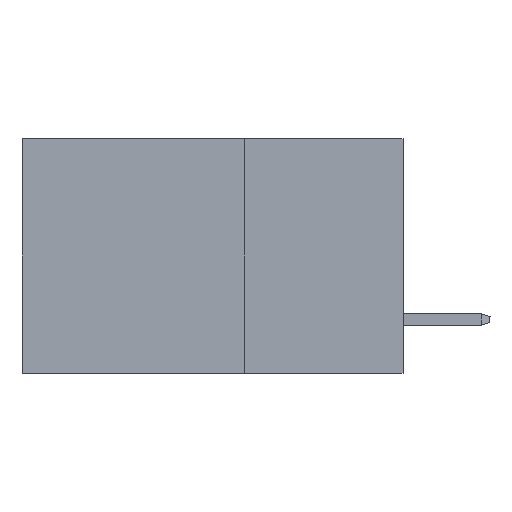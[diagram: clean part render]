
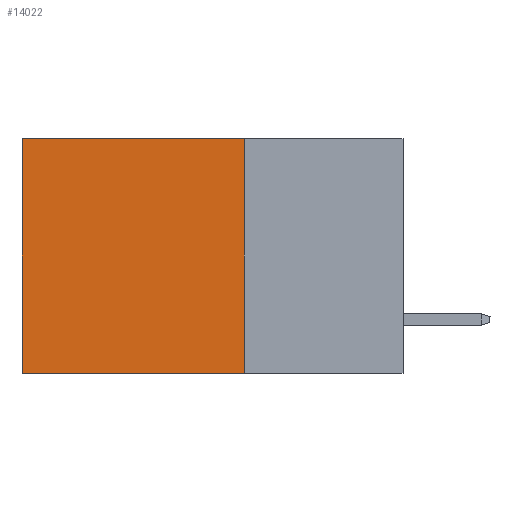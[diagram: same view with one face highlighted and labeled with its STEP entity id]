
A CAD part, left-side view. The second image highlights one B-rep face of the part: STEP entity #14022.
In plain terms, the highlighted planar face has unit normal (-1, 0, 0).
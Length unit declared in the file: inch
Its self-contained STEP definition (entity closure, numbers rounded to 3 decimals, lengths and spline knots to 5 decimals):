
#527 = VERTEX_POINT ( 'NONE', #16638 ) ;
#1776 = DIRECTION ( 'NONE',  ( 0., 0., -1. ) ) ;
#2168 = CARTESIAN_POINT ( 'NONE',  ( 0.2875, 0.6, 0. ) ) ;
#2653 = CARTESIAN_POINT ( 'NONE',  ( 0.2875, 0.25, 0. ) ) ;
#3952 = ORIENTED_EDGE ( 'NONE', *, *, #23253, .T. ) ;
#4387 = LINE ( 'NONE', #16398, #15092 ) ;
#6721 = DIRECTION ( 'NONE',  ( 1., 0., 0. ) ) ;
#6731 = DIRECTION ( 'NONE',  ( 0., 1., 0. ) ) ;
#7143 = DIRECTION ( 'NONE',  ( 0., 0., -1. ) ) ;
#7226 = CARTESIAN_POINT ( 'NONE',  ( 0.2875, 0.6, 0. ) ) ;
#8876 = LINE ( 'NONE', #11302, #16537 ) ;
#9631 = VECTOR ( 'NONE', #7143, 39.37008 ) ;
#9866 = EDGE_LOOP ( 'NONE', ( #25631, #18511, #17107, #3952 ) ) ;
#10125 = VECTOR ( 'NONE', #1776, 39.37008 ) ;
#11302 = CARTESIAN_POINT ( 'NONE',  ( 0.2875, 0.25, 0. ) ) ;
#11912 = VERTEX_POINT ( 'NONE', #24446 ) ;
#12943 = LINE ( 'NONE', #23744, #9631 ) ;
#13485 = EDGE_CURVE ( 'NONE', #18380, #527, #12943, .T. ) ;
#14022 = ADVANCED_FACE ( 'NONE', ( #25345 ), #16973, .F. ) ;
#14472 = LINE ( 'NONE', #2168, #10125 ) ;
#14944 = DIRECTION ( 'NONE',  ( 0., 0., -1. ) ) ;
#15092 = VECTOR ( 'NONE', #20857, 39.37008 ) ;
#15311 = AXIS2_PLACEMENT_3D ( 'NONE', #2653, #6721, #14944 ) ;
#16398 = CARTESIAN_POINT ( 'NONE',  ( 0.2875, 0.25, -0.37 ) ) ;
#16537 = VECTOR ( 'NONE', #6731, 39.37008 ) ;
#16638 = CARTESIAN_POINT ( 'NONE',  ( 0.2875, 0.25, -0.37 ) ) ;
#16973 = PLANE ( 'NONE',  #15311 ) ;
#17107 = ORIENTED_EDGE ( 'NONE', *, *, #13485, .F. ) ;
#17742 = EDGE_CURVE ( 'NONE', #527, #11912, #4387, .T. ) ;
#18380 = VERTEX_POINT ( 'NONE', #21088 ) ;
#18511 = ORIENTED_EDGE ( 'NONE', *, *, #17742, .F. ) ;
#20857 = DIRECTION ( 'NONE',  ( 0., 1., 0. ) ) ;
#21088 = CARTESIAN_POINT ( 'NONE',  ( 0.2875, 0.25, 0. ) ) ;
#23253 = EDGE_CURVE ( 'NONE', #18380, #26711, #8876, .T. ) ;
#23744 = CARTESIAN_POINT ( 'NONE',  ( 0.2875, 0.25, 0. ) ) ;
#24426 = EDGE_CURVE ( 'NONE', #26711, #11912, #14472, .T. ) ;
#24446 = CARTESIAN_POINT ( 'NONE',  ( 0.2875, 0.6, -0.37 ) ) ;
#25345 = FACE_OUTER_BOUND ( 'NONE', #9866, .T. ) ;
#25631 = ORIENTED_EDGE ( 'NONE', *, *, #24426, .T. ) ;
#26711 = VERTEX_POINT ( 'NONE', #7226 ) ;
